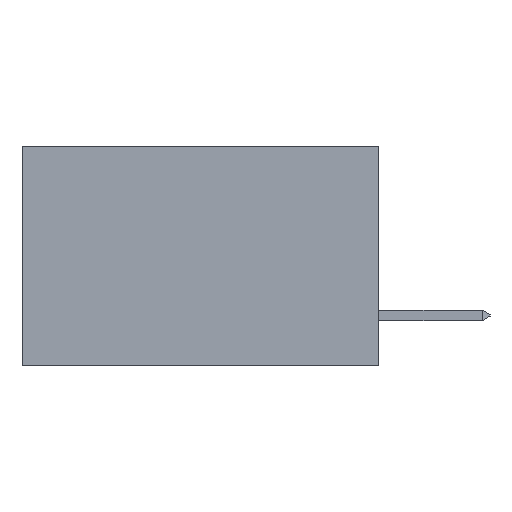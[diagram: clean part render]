
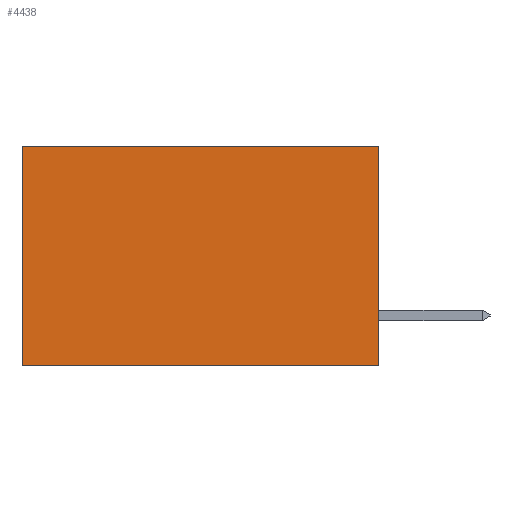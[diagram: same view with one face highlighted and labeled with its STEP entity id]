
A CAD part, left-side view. The second image highlights one B-rep face of the part: STEP entity #4438.
In plain terms, the highlighted planar face has unit normal (-1, 0, 0).
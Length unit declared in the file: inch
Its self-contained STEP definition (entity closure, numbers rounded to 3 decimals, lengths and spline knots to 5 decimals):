
#50 = DIRECTION ( 'NONE',  ( 1., 0., 0. ) ) ;
#79 = CARTESIAN_POINT ( 'NONE',  ( 0.2615, 0., -0.37 ) ) ;
#100 = PLANE ( 'NONE',  #10213 ) ;
#478 = ORIENTED_EDGE ( 'NONE', *, *, #1969, .T. ) ;
#1673 = DIRECTION ( 'NONE',  ( 0., 1., 0. ) ) ;
#1754 = CARTESIAN_POINT ( 'NONE',  ( 0.2615, 0., -0.37 ) ) ;
#1969 = EDGE_CURVE ( 'NONE', #7822, #11791, #12729, .T. ) ;
#2213 = VECTOR ( 'NONE', #24349, 39.37008 ) ;
#4438 = ADVANCED_FACE ( 'NONE', ( #6679 ), #100, .F. ) ;
#5832 = VECTOR ( 'NONE', #19605, 39.37008 ) ;
#6273 = VERTEX_POINT ( 'NONE', #1754 ) ;
#6679 = FACE_OUTER_BOUND ( 'NONE', #15770, .T. ) ;
#7189 = DIRECTION ( 'NONE',  ( 0., 0., -1. ) ) ;
#7663 = VECTOR ( 'NONE', #21544, 39.37008 ) ;
#7822 = VERTEX_POINT ( 'NONE', #18822 ) ;
#8829 = LINE ( 'NONE', #20770, #23260 ) ;
#9069 = ORIENTED_EDGE ( 'NONE', *, *, #18731, .T. ) ;
#10213 = AXIS2_PLACEMENT_3D ( 'NONE', #79, #50, #7189 ) ;
#11285 = CARTESIAN_POINT ( 'NONE',  ( 0.2615, 0., -0.37 ) ) ;
#11791 = VERTEX_POINT ( 'NONE', #22886 ) ;
#12127 = EDGE_CURVE ( 'NONE', #6273, #11791, #21599, .T. ) ;
#12729 = LINE ( 'NONE', #18025, #7663 ) ;
#14375 = ORIENTED_EDGE ( 'NONE', *, *, #23858, .F. ) ;
#15252 = ORIENTED_EDGE ( 'NONE', *, *, #12127, .F. ) ;
#15770 = EDGE_LOOP ( 'NONE', ( #478, #15252, #14375, #9069 ) ) ;
#16952 = LINE ( 'NONE', #11285, #2213 ) ;
#17618 = CARTESIAN_POINT ( 'NONE',  ( 0.2615, 0., 0. ) ) ;
#18025 = CARTESIAN_POINT ( 'NONE',  ( 0.2615, 0.6, -0.37 ) ) ;
#18731 = EDGE_CURVE ( 'NONE', #24103, #7822, #8829, .T. ) ;
#18822 = CARTESIAN_POINT ( 'NONE',  ( 0.2615, 0.6, 0. ) ) ;
#19462 = CARTESIAN_POINT ( 'NONE',  ( 0.2615, 0., -0.37 ) ) ;
#19605 = DIRECTION ( 'NONE',  ( 0., 1., 0. ) ) ;
#20770 = CARTESIAN_POINT ( 'NONE',  ( 0.2615, 0., 0. ) ) ;
#21544 = DIRECTION ( 'NONE',  ( 0., 0., -1. ) ) ;
#21599 = LINE ( 'NONE', #19462, #5832 ) ;
#22886 = CARTESIAN_POINT ( 'NONE',  ( 0.2615, 0.6, -0.37 ) ) ;
#23260 = VECTOR ( 'NONE', #1673, 39.37008 ) ;
#23858 = EDGE_CURVE ( 'NONE', #24103, #6273, #16952, .T. ) ;
#24103 = VERTEX_POINT ( 'NONE', #17618 ) ;
#24349 = DIRECTION ( 'NONE',  ( 0., 0., -1. ) ) ;
